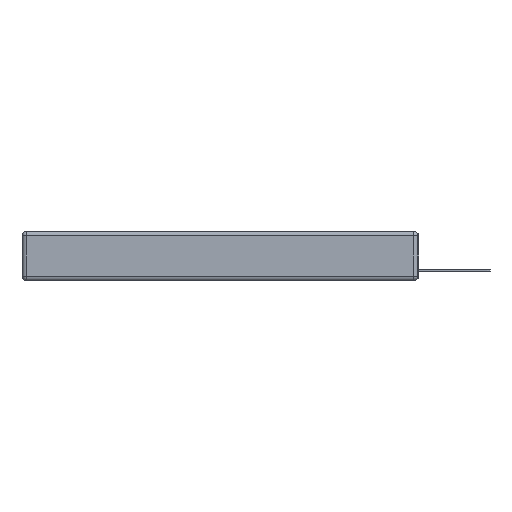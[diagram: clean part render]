
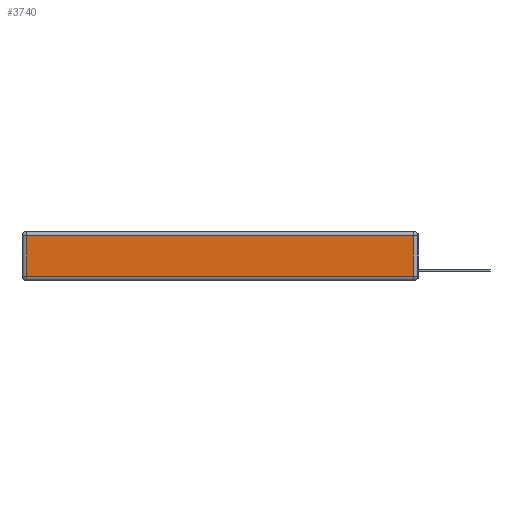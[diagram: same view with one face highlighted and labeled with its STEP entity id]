
A CAD part, left-side view. The second image highlights one B-rep face of the part: STEP entity #3740.
In plain terms, the highlighted planar face has unit normal (-1, 0, 0).
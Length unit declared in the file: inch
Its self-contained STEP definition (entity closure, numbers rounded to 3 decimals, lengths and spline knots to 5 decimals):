
#882 = CARTESIAN_POINT ( 'NONE',  ( 0., 0.03, -0.343 ) ) ;
#1960 = VERTEX_POINT ( 'NONE', #5297 ) ;
#2410 = CARTESIAN_POINT ( 'NONE',  ( 0., 2.72, -0.03 ) ) ;
#2494 = CARTESIAN_POINT ( 'NONE',  ( 0., 2.75, -0.03 ) ) ;
#2696 = CARTESIAN_POINT ( 'NONE',  ( 0., 0.03, -0.313 ) ) ;
#3075 = CARTESIAN_POINT ( 'NONE',  ( 0., 0., -0.313 ) ) ;
#3360 = ORIENTED_EDGE ( 'NONE', *, *, #25201, .T. ) ;
#3572 = DIRECTION ( 'NONE',  ( -1., 0., 0. ) ) ;
#3740 = ADVANCED_FACE ( 'NONE', ( #6879 ), #19714, .T. ) ;
#4031 = CARTESIAN_POINT ( 'NONE',  ( 0., 2.72, -0.313 ) ) ;
#5297 = CARTESIAN_POINT ( 'NONE',  ( 0., 0.03, -0.03 ) ) ;
#5606 = VECTOR ( 'NONE', #7289, 39.37008 ) ;
#5901 = ORIENTED_EDGE ( 'NONE', *, *, #17400, .T. ) ;
#6272 = VECTOR ( 'NONE', #16700, 39.37008 ) ;
#6531 = LINE ( 'NONE', #3075, #5606 ) ;
#6879 = FACE_OUTER_BOUND ( 'NONE', #14337, .T. ) ;
#6909 = LINE ( 'NONE', #2494, #6272 ) ;
#7289 = DIRECTION ( 'NONE',  ( 0., -1., 0. ) ) ;
#7743 = EDGE_CURVE ( 'NONE', #1960, #10263, #6909, .T. ) ;
#8597 = DIRECTION ( 'NONE',  ( 0., 0., -1. ) ) ;
#9860 = ORIENTED_EDGE ( 'NONE', *, *, #7743, .T. ) ;
#10263 = VERTEX_POINT ( 'NONE', #2410 ) ;
#11357 = VECTOR ( 'NONE', #8597, 39.37008 ) ;
#12702 = AXIS2_PLACEMENT_3D ( 'NONE', #25739, #3572, #18024 ) ;
#13599 = LINE ( 'NONE', #882, #23722 ) ;
#14337 = EDGE_LOOP ( 'NONE', ( #5901, #3360, #9860, #20857 ) ) ;
#14545 = CARTESIAN_POINT ( 'NONE',  ( 0., 2.72, -0.343 ) ) ;
#16700 = DIRECTION ( 'NONE',  ( 0., 1., 0. ) ) ;
#17400 = EDGE_CURVE ( 'NONE', #24125, #21960, #6531, .T. ) ;
#18024 = DIRECTION ( 'NONE',  ( 0., 0., 1. ) ) ;
#19714 = PLANE ( 'NONE',  #12702 ) ;
#20857 = ORIENTED_EDGE ( 'NONE', *, *, #22460, .T. ) ;
#21828 = LINE ( 'NONE', #14545, #11357 ) ;
#21960 = VERTEX_POINT ( 'NONE', #2696 ) ;
#22460 = EDGE_CURVE ( 'NONE', #10263, #24125, #21828, .T. ) ;
#23722 = VECTOR ( 'NONE', #25307, 39.37008 ) ;
#24125 = VERTEX_POINT ( 'NONE', #4031 ) ;
#25201 = EDGE_CURVE ( 'NONE', #21960, #1960, #13599, .T. ) ;
#25307 = DIRECTION ( 'NONE',  ( 0., 0., 1. ) ) ;
#25739 = CARTESIAN_POINT ( 'NONE',  ( 0., 0., -0.343 ) ) ;
